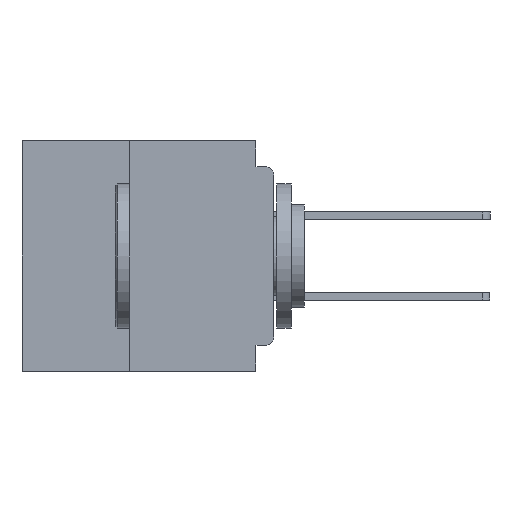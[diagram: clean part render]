
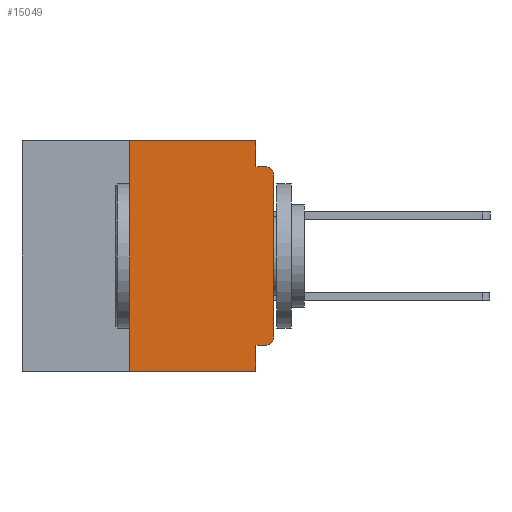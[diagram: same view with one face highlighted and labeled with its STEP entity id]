
A CAD part, left-side view. The second image highlights one B-rep face of the part: STEP entity #15049.
In plain terms, the highlighted planar face has unit normal (-1, 0, 0).
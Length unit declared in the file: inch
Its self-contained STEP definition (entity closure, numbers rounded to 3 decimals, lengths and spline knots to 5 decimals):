
#2208 = CARTESIAN_POINT ( 'NONE',  ( 0., 0.031, 0. ) ) ;
#2732 = ORIENTED_EDGE ( 'NONE', *, *, #25208, .T. ) ;
#3167 = CARTESIAN_POINT ( 'NONE',  ( 0., 0.031, -0.4 ) ) ;
#3626 = EDGE_CURVE ( 'NONE', #26323, #12554, #5421, .T. ) ;
#5389 = CARTESIAN_POINT ( 'NONE',  ( 0., 0., -0.34 ) ) ;
#5421 = CIRCLE ( 'NONE', #32761, 0.015 ) ;
#5519 = ORIENTED_EDGE ( 'NONE', *, *, #3626, .T. ) ;
#5715 = VECTOR ( 'NONE', #7239, 39.37008 ) ;
#5887 = CARTESIAN_POINT ( 'NONE',  ( 0., 0.437, 0. ) ) ;
#6210 = DIRECTION ( 'NONE',  ( 0., 0., -1. ) ) ;
#6246 = DIRECTION ( 'NONE',  ( -1., 0., 0. ) ) ;
#6258 = CARTESIAN_POINT ( 'NONE',  ( 0., 0.015, -0.06 ) ) ;
#7239 = DIRECTION ( 'NONE',  ( 0., -1., 0. ) ) ;
#7321 = LINE ( 'NONE', #16306, #42506 ) ;
#7640 = ORIENTED_EDGE ( 'NONE', *, *, #38651, .T. ) ;
#7882 = EDGE_CURVE ( 'NONE', #41779, #9226, #39301, .T. ) ;
#8388 = DIRECTION ( 'NONE',  ( 0., 0., 1. ) ) ;
#9226 = VERTEX_POINT ( 'NONE', #5389 ) ;
#9374 = DIRECTION ( 'NONE',  ( 0., 0., -1. ) ) ;
#9780 = EDGE_CURVE ( 'NONE', #24084, #41049, #36975, .T. ) ;
#10036 = ORIENTED_EDGE ( 'NONE', *, *, #23916, .F. ) ;
#10092 = LINE ( 'NONE', #20444, #19209 ) ;
#10581 = AXIS2_PLACEMENT_3D ( 'NONE', #16042, #39884, #19471 ) ;
#11498 = VECTOR ( 'NONE', #34961, 39.37008 ) ;
#11975 = CARTESIAN_POINT ( 'NONE',  ( 0., 0.031, -0.4 ) ) ;
#12393 = LINE ( 'NONE', #24098, #28477 ) ;
#12554 = VERTEX_POINT ( 'NONE', #14551 ) ;
#13556 = VECTOR ( 'NONE', #43604, 39.37008 ) ;
#14551 = CARTESIAN_POINT ( 'NONE',  ( 0., 0.015, -0.045 ) ) ;
#15049 = ADVANCED_FACE ( 'NONE', ( #39205 ), #26452, .F. ) ;
#15054 = VERTEX_POINT ( 'NONE', #2208 ) ;
#15498 = VERTEX_POINT ( 'NONE', #28680 ) ;
#16042 = CARTESIAN_POINT ( 'NONE',  ( 0., 0.015, -0.34 ) ) ;
#16306 = CARTESIAN_POINT ( 'NONE',  ( 0., 0.437, -0.4 ) ) ;
#16904 = ORIENTED_EDGE ( 'NONE', *, *, #20561, .F. ) ;
#19209 = VECTOR ( 'NONE', #44217, 39.37008 ) ;
#19471 = DIRECTION ( 'NONE',  ( 0., 0., -1. ) ) ;
#19554 = VERTEX_POINT ( 'NONE', #41968 ) ;
#19834 = CARTESIAN_POINT ( 'NONE',  ( 0., 0., -0.355 ) ) ;
#20254 = CARTESIAN_POINT ( 'NONE',  ( 0., 0., -0.06 ) ) ;
#20444 = CARTESIAN_POINT ( 'NONE',  ( 0., 0., 0. ) ) ;
#20561 = EDGE_CURVE ( 'NONE', #15498, #15054, #33075, .T. ) ;
#20565 = CARTESIAN_POINT ( 'NONE',  ( 0., 0.031, -0.355 ) ) ;
#22653 = LINE ( 'NONE', #19834, #13556 ) ;
#22728 = LINE ( 'NONE', #38360, #11498 ) ;
#23916 = EDGE_CURVE ( 'NONE', #41779, #24084, #22653, .T. ) ;
#24084 = VERTEX_POINT ( 'NONE', #20565 ) ;
#24098 = CARTESIAN_POINT ( 'NONE',  ( 0., 0.031, 0. ) ) ;
#25208 = EDGE_CURVE ( 'NONE', #30366, #41049, #7321, .T. ) ;
#26323 = VERTEX_POINT ( 'NONE', #20254 ) ;
#26452 = PLANE ( 'NONE',  #30022 ) ;
#27031 = LINE ( 'NONE', #35705, #35010 ) ;
#28233 = ORIENTED_EDGE ( 'NONE', *, *, #29357, .F. ) ;
#28419 = CARTESIAN_POINT ( 'NONE',  ( 0., 0.015, -0.355 ) ) ;
#28477 = VECTOR ( 'NONE', #37636, 39.37008 ) ;
#28607 = EDGE_LOOP ( 'NONE', ( #7640, #5519, #37970, #28233, #16904, #34596, #2732, #31629, #10036, #39615 ) ) ;
#28680 = CARTESIAN_POINT ( 'NONE',  ( 0., 0.25, 0. ) ) ;
#29357 = EDGE_CURVE ( 'NONE', #15054, #19554, #12393, .T. ) ;
#29905 = DIRECTION ( 'NONE',  ( 1., 0., 0. ) ) ;
#30022 = AXIS2_PLACEMENT_3D ( 'NONE', #5887, #29905, #9374 ) ;
#30366 = VERTEX_POINT ( 'NONE', #43593 ) ;
#31225 = CARTESIAN_POINT ( 'NONE',  ( 0., 0.437, 0. ) ) ;
#31424 = EDGE_CURVE ( 'NONE', #30366, #15498, #27031, .T. ) ;
#31564 = EDGE_CURVE ( 'NONE', #19554, #12554, #22728, .T. ) ;
#31629 = ORIENTED_EDGE ( 'NONE', *, *, #9780, .F. ) ;
#32761 = AXIS2_PLACEMENT_3D ( 'NONE', #6258, #6246, #6210 ) ;
#32776 = VECTOR ( 'NONE', #39271, 39.37008 ) ;
#33075 = LINE ( 'NONE', #31225, #5715 ) ;
#34596 = ORIENTED_EDGE ( 'NONE', *, *, #31424, .F. ) ;
#34961 = DIRECTION ( 'NONE',  ( 0., -1., 0. ) ) ;
#35010 = VECTOR ( 'NONE', #8388, 39.37008 ) ;
#35705 = CARTESIAN_POINT ( 'NONE',  ( 0., 0.25, -0.4 ) ) ;
#36975 = LINE ( 'NONE', #11975, #32776 ) ;
#37636 = DIRECTION ( 'NONE',  ( 0., 0., -1. ) ) ;
#37970 = ORIENTED_EDGE ( 'NONE', *, *, #31564, .F. ) ;
#38360 = CARTESIAN_POINT ( 'NONE',  ( 0., 0., -0.045 ) ) ;
#38651 = EDGE_CURVE ( 'NONE', #9226, #26323, #10092, .T. ) ;
#39205 = FACE_OUTER_BOUND ( 'NONE', #28607, .T. ) ;
#39271 = DIRECTION ( 'NONE',  ( 0., 0., -1. ) ) ;
#39301 = CIRCLE ( 'NONE', #10581, 0.015 ) ;
#39615 = ORIENTED_EDGE ( 'NONE', *, *, #7882, .T. ) ;
#39884 = DIRECTION ( 'NONE',  ( -1., 0., 0. ) ) ;
#40149 = DIRECTION ( 'NONE',  ( 0., -1., 0. ) ) ;
#41049 = VERTEX_POINT ( 'NONE', #3167 ) ;
#41779 = VERTEX_POINT ( 'NONE', #28419 ) ;
#41968 = CARTESIAN_POINT ( 'NONE',  ( 0., 0.031, -0.045 ) ) ;
#42506 = VECTOR ( 'NONE', #40149, 39.37008 ) ;
#43593 = CARTESIAN_POINT ( 'NONE',  ( 0., 0.25, -0.4 ) ) ;
#43604 = DIRECTION ( 'NONE',  ( 0., 1., 0. ) ) ;
#44217 = DIRECTION ( 'NONE',  ( 0., 0., 1. ) ) ;
